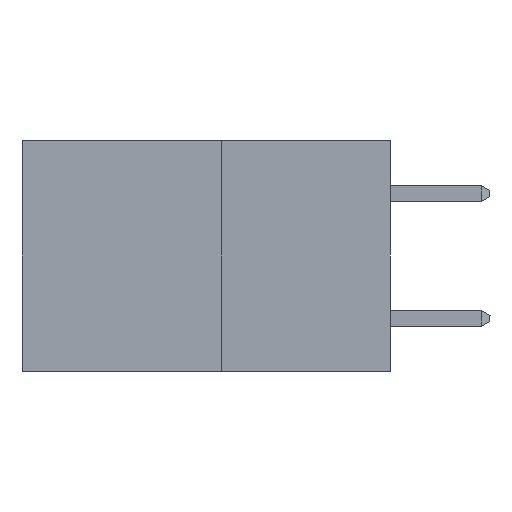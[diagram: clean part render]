
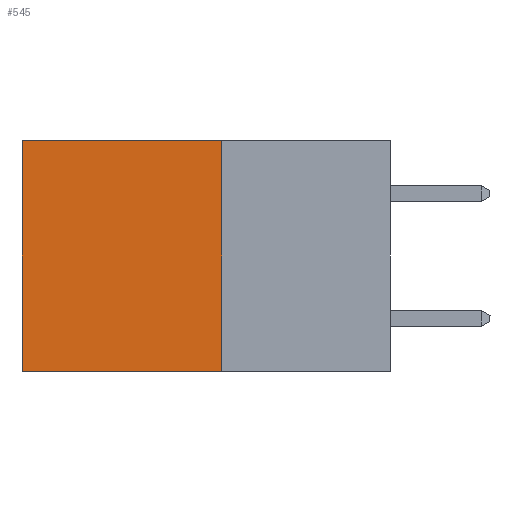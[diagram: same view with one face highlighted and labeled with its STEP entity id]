
A CAD part, left-side view. The second image highlights one B-rep face of the part: STEP entity #545.
In plain terms, the highlighted planar face has unit normal (-1, 0, 0).
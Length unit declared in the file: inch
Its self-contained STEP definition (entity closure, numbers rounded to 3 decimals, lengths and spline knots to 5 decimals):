
#380 = DIRECTION ( 'NONE',  ( 0., 1., 0. ) ) ;
#545 = ADVANCED_FACE ( 'NONE', ( #8348 ), #3792, .F. ) ;
#952 = LINE ( 'NONE', #11963, #5516 ) ;
#1558 = CARTESIAN_POINT ( 'NONE',  ( 0.277, 0.59, 0. ) ) ;
#1593 = VECTOR ( 'NONE', #10421, 39.37008 ) ;
#1880 = VERTEX_POINT ( 'NONE', #10433 ) ;
#3262 = ORIENTED_EDGE ( 'NONE', *, *, #5617, .F. ) ;
#3703 = EDGE_CURVE ( 'NONE', #9149, #5382, #11301, .T. ) ;
#3792 = PLANE ( 'NONE',  #6794 ) ;
#3834 = DIRECTION ( 'NONE',  ( 0., 0., -1. ) ) ;
#4150 = CARTESIAN_POINT ( 'NONE',  ( 0.277, 0.59, -0.37 ) ) ;
#4648 = EDGE_LOOP ( 'NONE', ( #4805, #6725, #3262, #6208 ) ) ;
#4805 = ORIENTED_EDGE ( 'NONE', *, *, #3703, .T. ) ;
#4990 = CARTESIAN_POINT ( 'NONE',  ( 0.277, 0.27, 0. ) ) ;
#5326 = DIRECTION ( 'NONE',  ( 1., 0., 0. ) ) ;
#5382 = VERTEX_POINT ( 'NONE', #4150 ) ;
#5516 = VECTOR ( 'NONE', #380, 39.37008 ) ;
#5617 = EDGE_CURVE ( 'NONE', #1880, #10052, #10024, .T. ) ;
#5963 = DIRECTION ( 'NONE',  ( 0., 1., 0. ) ) ;
#6208 = ORIENTED_EDGE ( 'NONE', *, *, #12443, .T. ) ;
#6725 = ORIENTED_EDGE ( 'NONE', *, *, #8971, .F. ) ;
#6794 = AXIS2_PLACEMENT_3D ( 'NONE', #12515, #5326, #3834 ) ;
#7379 = VECTOR ( 'NONE', #5963, 39.37008 ) ;
#7826 = CARTESIAN_POINT ( 'NONE',  ( 0.277, 0.27, -0.37 ) ) ;
#8348 = FACE_OUTER_BOUND ( 'NONE', #4648, .T. ) ;
#8971 = EDGE_CURVE ( 'NONE', #10052, #5382, #952, .T. ) ;
#9149 = VERTEX_POINT ( 'NONE', #1558 ) ;
#9689 = CARTESIAN_POINT ( 'NONE',  ( 0.277, 0.59, -0.37 ) ) ;
#10024 = LINE ( 'NONE', #12123, #12287 ) ;
#10052 = VERTEX_POINT ( 'NONE', #7826 ) ;
#10421 = DIRECTION ( 'NONE',  ( 0., 0., -1. ) ) ;
#10433 = CARTESIAN_POINT ( 'NONE',  ( 0.277, 0.27, 0. ) ) ;
#10572 = LINE ( 'NONE', #4990, #7379 ) ;
#11301 = LINE ( 'NONE', #9689, #1593 ) ;
#11963 = CARTESIAN_POINT ( 'NONE',  ( 0.277, 0.27, -0.37 ) ) ;
#12042 = DIRECTION ( 'NONE',  ( 0., 0., -1. ) ) ;
#12123 = CARTESIAN_POINT ( 'NONE',  ( 0.277, 0.27, -0.37 ) ) ;
#12287 = VECTOR ( 'NONE', #12042, 39.37008 ) ;
#12443 = EDGE_CURVE ( 'NONE', #1880, #9149, #10572, .T. ) ;
#12515 = CARTESIAN_POINT ( 'NONE',  ( 0.277, 0.27, -0.37 ) ) ;
